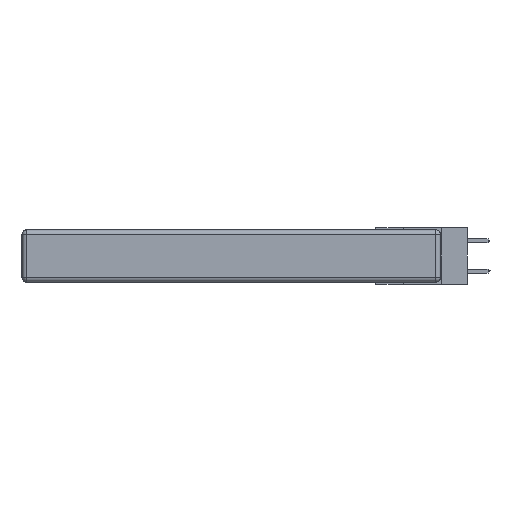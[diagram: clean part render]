
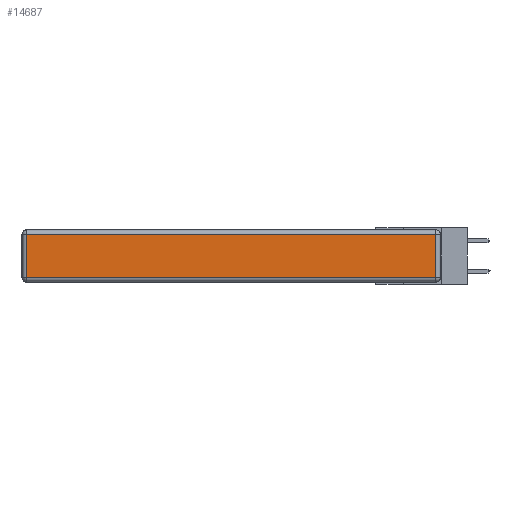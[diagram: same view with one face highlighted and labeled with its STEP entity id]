
A CAD part, left-side view. The second image highlights one B-rep face of the part: STEP entity #14687.
In plain terms, the highlighted planar face has unit normal (-1, 0, 0).
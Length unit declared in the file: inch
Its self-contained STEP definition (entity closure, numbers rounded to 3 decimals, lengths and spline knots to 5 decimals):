
#480 = DIRECTION ( 'NONE',  ( 0., 1., 0. ) ) ;
#1384 = LINE ( 'NONE', #8013, #13141 ) ;
#2184 = DIRECTION ( 'NONE',  ( 0., 0., -1. ) ) ;
#2814 = FACE_OUTER_BOUND ( 'NONE', #9826, .T. ) ;
#2971 = CARTESIAN_POINT ( 'NONE',  ( 0., 0.03, -0.313 ) ) ;
#3415 = EDGE_CURVE ( 'NONE', #17214, #4436, #5510, .T. ) ;
#3579 = EDGE_CURVE ( 'NONE', #11993, #8740, #9663, .T. ) ;
#4345 = ORIENTED_EDGE ( 'NONE', *, *, #3415, .T. ) ;
#4436 = VERTEX_POINT ( 'NONE', #2971 ) ;
#4834 = ORIENTED_EDGE ( 'NONE', *, *, #13149, .T. ) ;
#4904 = EDGE_CURVE ( 'NONE', #4436, #11993, #1384, .T. ) ;
#5510 = LINE ( 'NONE', #13871, #8166 ) ;
#5664 = LINE ( 'NONE', #13512, #16349 ) ;
#5777 = CARTESIAN_POINT ( 'NONE',  ( 0., 0., -0.343 ) ) ;
#7267 = DIRECTION ( 'NONE',  ( 0., 0., 1. ) ) ;
#8013 = CARTESIAN_POINT ( 'NONE',  ( 0., 0.03, -0.343 ) ) ;
#8166 = VECTOR ( 'NONE', #17903, 39.37008 ) ;
#8549 = PLANE ( 'NONE',  #11446 ) ;
#8740 = VERTEX_POINT ( 'NONE', #12345 ) ;
#8834 = CARTESIAN_POINT ( 'NONE',  ( 0., 0.03, -0.03 ) ) ;
#9489 = ORIENTED_EDGE ( 'NONE', *, *, #4904, .T. ) ;
#9663 = LINE ( 'NONE', #14418, #11431 ) ;
#9826 = EDGE_LOOP ( 'NONE', ( #4345, #9489, #12558, #4834 ) ) ;
#10035 = CARTESIAN_POINT ( 'NONE',  ( 0., 2.72, -0.313 ) ) ;
#10931 = DIRECTION ( 'NONE',  ( 0., 0., 1. ) ) ;
#11431 = VECTOR ( 'NONE', #480, 39.37008 ) ;
#11446 = AXIS2_PLACEMENT_3D ( 'NONE', #5777, #15531, #7267 ) ;
#11993 = VERTEX_POINT ( 'NONE', #8834 ) ;
#12345 = CARTESIAN_POINT ( 'NONE',  ( 0., 2.72, -0.03 ) ) ;
#12558 = ORIENTED_EDGE ( 'NONE', *, *, #3579, .T. ) ;
#13141 = VECTOR ( 'NONE', #10931, 39.37008 ) ;
#13149 = EDGE_CURVE ( 'NONE', #8740, #17214, #5664, .T. ) ;
#13512 = CARTESIAN_POINT ( 'NONE',  ( 0., 2.72, -0.343 ) ) ;
#13871 = CARTESIAN_POINT ( 'NONE',  ( 0., 0., -0.313 ) ) ;
#14418 = CARTESIAN_POINT ( 'NONE',  ( 0., 2.75, -0.03 ) ) ;
#14687 = ADVANCED_FACE ( 'NONE', ( #2814 ), #8549, .T. ) ;
#15531 = DIRECTION ( 'NONE',  ( -1., 0., 0. ) ) ;
#16349 = VECTOR ( 'NONE', #2184, 39.37008 ) ;
#17214 = VERTEX_POINT ( 'NONE', #10035 ) ;
#17903 = DIRECTION ( 'NONE',  ( 0., -1., 0. ) ) ;
